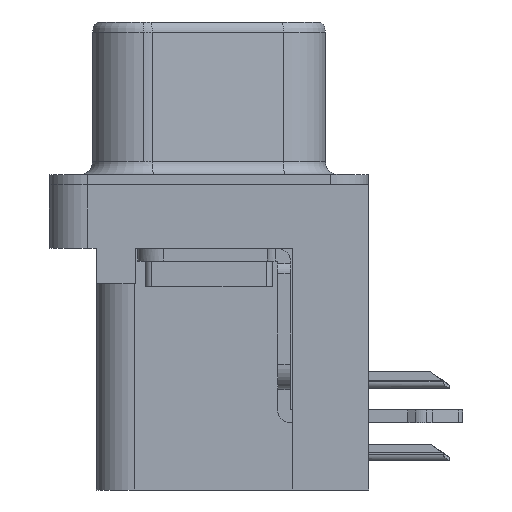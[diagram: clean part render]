
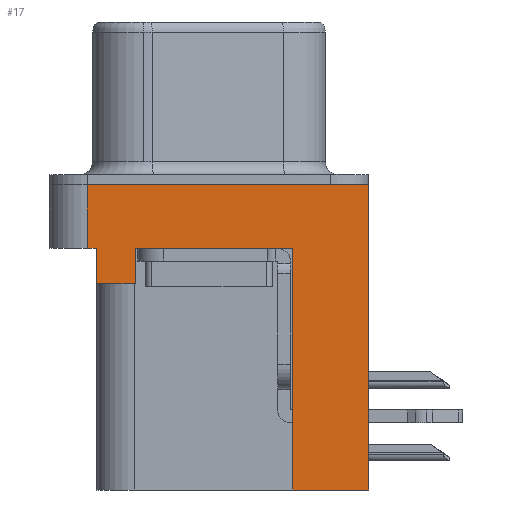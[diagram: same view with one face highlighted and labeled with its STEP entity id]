
A CAD part, left-side view. The second image highlights one B-rep face of the part: STEP entity #17.
In plain terms, the highlighted planar face has unit normal (-1, 0, 0).
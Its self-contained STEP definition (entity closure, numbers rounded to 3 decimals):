
#17 = ADVANCED_FACE ( 'NONE', ( #20161 ), #9109, .T. ) ;
#767 = CARTESIAN_POINT ( 'NONE',  ( -3., -3.295, -2.5 ) ) ;
#1269 = CARTESIAN_POINT ( 'NONE',  ( -3., -3.295, -12. ) ) ;
#2129 = ORIENTED_EDGE ( 'NONE', *, *, #11921, .T. ) ;
#2148 = ORIENTED_EDGE ( 'NONE', *, *, #9739, .F. ) ;
#2209 = LINE ( 'NONE', #17737, #21634 ) ;
#2675 = CARTESIAN_POINT ( 'NONE',  ( -3., 4.425, -3.9 ) ) ;
#2986 = CARTESIAN_POINT ( 'NONE',  ( -3., -6.275, -2.5 ) ) ;
#3482 = VECTOR ( 'NONE', #10982, 1000. ) ;
#3741 = DIRECTION ( 'NONE',  ( -1., 0., 0. ) ) ;
#3838 = VERTEX_POINT ( 'NONE', #5726 ) ;
#3905 = VERTEX_POINT ( 'NONE', #19039 ) ;
#4030 = VERTEX_POINT ( 'NONE', #17198 ) ;
#4176 = VECTOR ( 'NONE', #17019, 1000. ) ;
#4502 = ORIENTED_EDGE ( 'NONE', *, *, #11643, .F. ) ;
#4881 = DIRECTION ( 'NONE',  ( 0., -1., 0. ) ) ;
#5399 = VERTEX_POINT ( 'NONE', #12001 ) ;
#5478 = ORIENTED_EDGE ( 'NONE', *, *, #19607, .F. ) ;
#5561 = VECTOR ( 'NONE', #21113, 1000. ) ;
#5726 = CARTESIAN_POINT ( 'NONE',  ( -3., -3.295, -12. ) ) ;
#6793 = EDGE_CURVE ( 'NONE', #12819, #4030, #7540, .T. ) ;
#6839 = DIRECTION ( 'NONE',  ( 0., -1., 0. ) ) ;
#6955 = CARTESIAN_POINT ( 'NONE',  ( -3., 2.895, -2.5 ) ) ;
#7540 = LINE ( 'NONE', #10505, #10622 ) ;
#7600 = LINE ( 'NONE', #9469, #9020 ) ;
#7839 = VERTEX_POINT ( 'NONE', #6955 ) ;
#8492 = DIRECTION ( 'NONE',  ( 0., 0., 1. ) ) ;
#8743 = ORIENTED_EDGE ( 'NONE', *, *, #11260, .T. ) ;
#9020 = VECTOR ( 'NONE', #22069, 1000. ) ;
#9109 = PLANE ( 'NONE',  #17530 ) ;
#9158 = LINE ( 'NONE', #10218, #22102 ) ;
#9469 = CARTESIAN_POINT ( 'NONE',  ( -3., 4.775, -2.5 ) ) ;
#9604 = ORIENTED_EDGE ( 'NONE', *, *, #15971, .T. ) ;
#9665 = CARTESIAN_POINT ( 'NONE',  ( -3., 2.895, -3.9 ) ) ;
#9739 = EDGE_CURVE ( 'NONE', #14226, #14841, #19300, .T. ) ;
#9967 = VECTOR ( 'NONE', #13331, 1000. ) ;
#10218 = CARTESIAN_POINT ( 'NONE',  ( -3., -6.275, -2.5 ) ) ;
#10505 = CARTESIAN_POINT ( 'NONE',  ( -3., -6.275, 0. ) ) ;
#10622 = VECTOR ( 'NONE', #14147, 1000. ) ;
#10982 = DIRECTION ( 'NONE',  ( 0., 1., 0. ) ) ;
#11260 = EDGE_CURVE ( 'NONE', #7839, #22836, #9158, .T. ) ;
#11643 = EDGE_CURVE ( 'NONE', #14841, #20810, #15340, .T. ) ;
#11921 = EDGE_CURVE ( 'NONE', #5399, #20810, #17587, .T. ) ;
#12001 = CARTESIAN_POINT ( 'NONE',  ( -3., 4.775, -2.5 ) ) ;
#12734 = CARTESIAN_POINT ( 'NONE',  ( -3., 4.425, -3.9 ) ) ;
#12819 = VERTEX_POINT ( 'NONE', #19601 ) ;
#13129 = VECTOR ( 'NONE', #22259, 1000. ) ;
#13331 = DIRECTION ( 'NONE',  ( 0., 0., 1. ) ) ;
#14147 = DIRECTION ( 'NONE',  ( 0., -1., 0. ) ) ;
#14226 = VERTEX_POINT ( 'NONE', #19174 ) ;
#14545 = CARTESIAN_POINT ( 'NONE',  ( -3., -6.275, -2.5 ) ) ;
#14773 = DIRECTION ( 'NONE',  ( 0., 0., 1. ) ) ;
#14841 = VERTEX_POINT ( 'NONE', #19365 ) ;
#15206 = EDGE_CURVE ( 'NONE', #5399, #12819, #7600, .T. ) ;
#15340 = LINE ( 'NONE', #2675, #9967 ) ;
#15442 = EDGE_LOOP ( 'NONE', ( #17868, #16187, #2129, #4502, #2148, #9604, #8743, #19715, #5478, #15947 ) ) ;
#15947 = ORIENTED_EDGE ( 'NONE', *, *, #21231, .T. ) ;
#15971 = EDGE_CURVE ( 'NONE', #14226, #7839, #19162, .T. ) ;
#16111 = EDGE_CURVE ( 'NONE', #3838, #22836, #2209, .T. ) ;
#16187 = ORIENTED_EDGE ( 'NONE', *, *, #15206, .F. ) ;
#16222 = LINE ( 'NONE', #18907, #13129 ) ;
#16443 = VECTOR ( 'NONE', #6839, 1000. ) ;
#17019 = DIRECTION ( 'NONE',  ( 0., 0., 1. ) ) ;
#17198 = CARTESIAN_POINT ( 'NONE',  ( -3., -6.275, 0. ) ) ;
#17530 = AXIS2_PLACEMENT_3D ( 'NONE', #14545, #3741, #14773 ) ;
#17587 = LINE ( 'NONE', #2986, #16443 ) ;
#17737 = CARTESIAN_POINT ( 'NONE',  ( -3., -3.295, -12. ) ) ;
#17868 = ORIENTED_EDGE ( 'NONE', *, *, #6793, .F. ) ;
#18026 = LINE ( 'NONE', #1269, #5561 ) ;
#18907 = CARTESIAN_POINT ( 'NONE',  ( -3., -6.275, -2.5 ) ) ;
#19039 = CARTESIAN_POINT ( 'NONE',  ( -3., -6.275, -12. ) ) ;
#19162 = LINE ( 'NONE', #9665, #4176 ) ;
#19174 = CARTESIAN_POINT ( 'NONE',  ( -3., 2.895, -3.9 ) ) ;
#19300 = LINE ( 'NONE', #12734, #3482 ) ;
#19365 = CARTESIAN_POINT ( 'NONE',  ( -3., 4.425, -3.9 ) ) ;
#19480 = CARTESIAN_POINT ( 'NONE',  ( -3., 4.425, -2.5 ) ) ;
#19601 = CARTESIAN_POINT ( 'NONE',  ( -3., 4.775, 0. ) ) ;
#19607 = EDGE_CURVE ( 'NONE', #3905, #3838, #18026, .T. ) ;
#19715 = ORIENTED_EDGE ( 'NONE', *, *, #16111, .F. ) ;
#20161 = FACE_OUTER_BOUND ( 'NONE', #15442, .T. ) ;
#20810 = VERTEX_POINT ( 'NONE', #19480 ) ;
#21113 = DIRECTION ( 'NONE',  ( 0., 1., 0. ) ) ;
#21231 = EDGE_CURVE ( 'NONE', #3905, #4030, #16222, .T. ) ;
#21634 = VECTOR ( 'NONE', #8492, 1000. ) ;
#22069 = DIRECTION ( 'NONE',  ( 0., 0., 1. ) ) ;
#22102 = VECTOR ( 'NONE', #4881, 1000. ) ;
#22259 = DIRECTION ( 'NONE',  ( 0., 0., 1. ) ) ;
#22836 = VERTEX_POINT ( 'NONE', #767 ) ;
